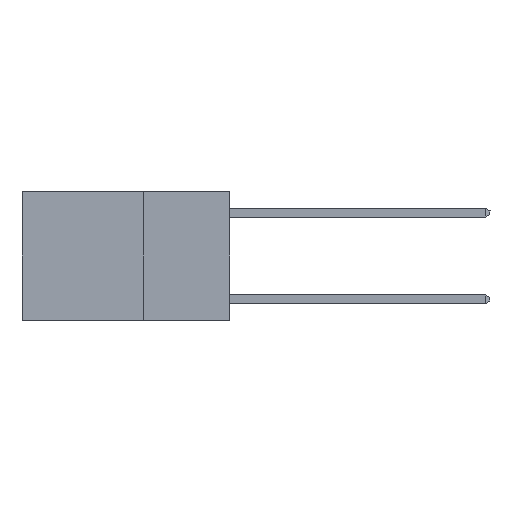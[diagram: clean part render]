
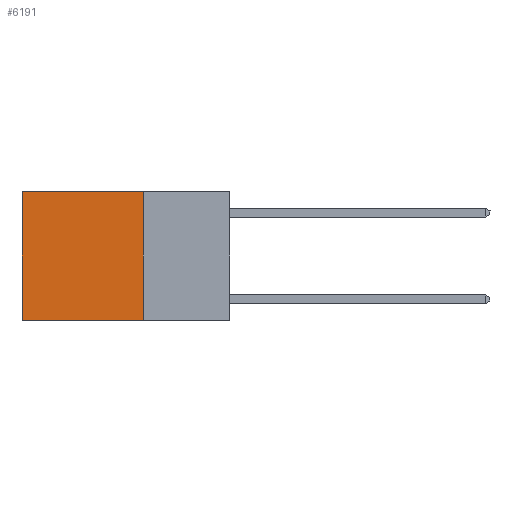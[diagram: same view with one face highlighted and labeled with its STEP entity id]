
A CAD part, left-side view. The second image highlights one B-rep face of the part: STEP entity #6191.
In plain terms, the highlighted planar face has unit normal (-1, 0, 0).
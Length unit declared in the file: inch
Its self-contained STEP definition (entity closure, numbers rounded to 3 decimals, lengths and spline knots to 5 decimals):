
#625 = ORIENTED_EDGE ( 'NONE', *, *, #25572, .T. ) ;
#1023 = CARTESIAN_POINT ( 'NONE',  ( 0.2625, 0.6, -0.37 ) ) ;
#1211 = CARTESIAN_POINT ( 'NONE',  ( 0.2625, 0.25, -0.37 ) ) ;
#1215 = CARTESIAN_POINT ( 'NONE',  ( 0.2625, 0.25, -0.37 ) ) ;
#1307 = DIRECTION ( 'NONE',  ( 0., 1., 0. ) ) ;
#3319 = AXIS2_PLACEMENT_3D ( 'NONE', #5150, #13177, #10906 ) ;
#3342 = LINE ( 'NONE', #21337, #22112 ) ;
#3625 = CARTESIAN_POINT ( 'NONE',  ( 0.2625, 0.25, 0. ) ) ;
#4459 = DIRECTION ( 'NONE',  ( 0., 0., -1. ) ) ;
#4614 = VERTEX_POINT ( 'NONE', #22349 ) ;
#5150 = CARTESIAN_POINT ( 'NONE',  ( 0.2625, 0.25, 0. ) ) ;
#5712 = ORIENTED_EDGE ( 'NONE', *, *, #17585, .F. ) ;
#5853 = DIRECTION ( 'NONE',  ( 0., 0., -1. ) ) ;
#6191 = ADVANCED_FACE ( 'NONE', ( #14200 ), #8899, .F. ) ;
#6235 = VERTEX_POINT ( 'NONE', #1023 ) ;
#7425 = ORIENTED_EDGE ( 'NONE', *, *, #9758, .T. ) ;
#8448 = VECTOR ( 'NONE', #5853, 39.37008 ) ;
#8478 = VECTOR ( 'NONE', #17289, 39.37008 ) ;
#8899 = PLANE ( 'NONE',  #3319 ) ;
#9758 = EDGE_CURVE ( 'NONE', #4614, #6235, #19212, .T. ) ;
#10236 = EDGE_LOOP ( 'NONE', ( #7425, #14915, #5712, #625 ) ) ;
#10565 = VERTEX_POINT ( 'NONE', #1211 ) ;
#10649 = LINE ( 'NONE', #1215, #8478 ) ;
#10773 = VECTOR ( 'NONE', #4459, 39.37008 ) ;
#10906 = DIRECTION ( 'NONE',  ( 0., 0., -1. ) ) ;
#12110 = EDGE_CURVE ( 'NONE', #10565, #6235, #10649, .T. ) ;
#13055 = VERTEX_POINT ( 'NONE', #3625 ) ;
#13177 = DIRECTION ( 'NONE',  ( 1., 0., 0. ) ) ;
#14200 = FACE_OUTER_BOUND ( 'NONE', #10236, .T. ) ;
#14915 = ORIENTED_EDGE ( 'NONE', *, *, #12110, .F. ) ;
#17163 = LINE ( 'NONE', #23779, #8448 ) ;
#17289 = DIRECTION ( 'NONE',  ( 0., 1., 0. ) ) ;
#17585 = EDGE_CURVE ( 'NONE', #13055, #10565, #17163, .T. ) ;
#19212 = LINE ( 'NONE', #20807, #10773 ) ;
#20807 = CARTESIAN_POINT ( 'NONE',  ( 0.2625, 0.6, 0. ) ) ;
#21337 = CARTESIAN_POINT ( 'NONE',  ( 0.2625, 0.25, 0. ) ) ;
#22112 = VECTOR ( 'NONE', #1307, 39.37008 ) ;
#22349 = CARTESIAN_POINT ( 'NONE',  ( 0.2625, 0.6, 0. ) ) ;
#23779 = CARTESIAN_POINT ( 'NONE',  ( 0.2625, 0.25, 0. ) ) ;
#25572 = EDGE_CURVE ( 'NONE', #13055, #4614, #3342, .T. ) ;
